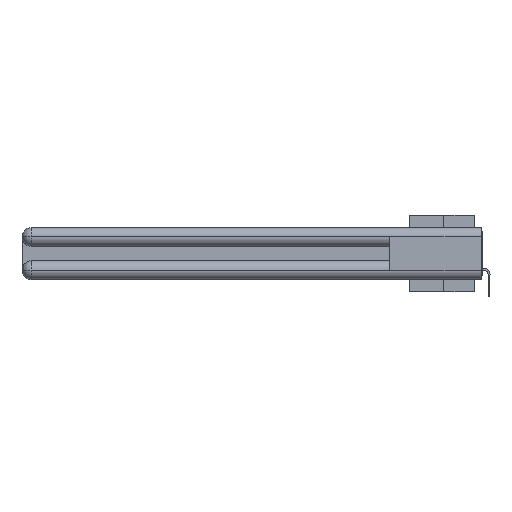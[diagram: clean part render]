
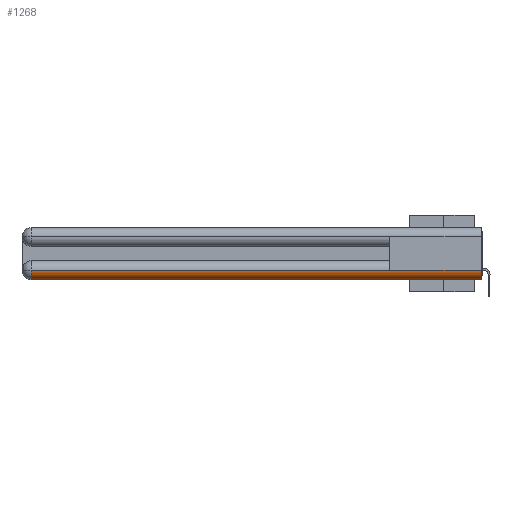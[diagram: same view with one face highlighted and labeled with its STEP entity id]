
A CAD part, left-side view. The second image highlights one B-rep face of the part: STEP entity #1268.
In plain terms, the highlighted cylindrical face has radius 1.562 mm (diameter 3.124 mm), a partial arc.
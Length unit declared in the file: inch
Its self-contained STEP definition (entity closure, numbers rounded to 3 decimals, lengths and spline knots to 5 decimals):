
#1268 = ADVANCED_FACE ( 'NONE', ( #8124 ), #1566, .T. ) ;
#1288 = CARTESIAN_POINT ( 'NONE',  ( 0.0615, 0., -0.2785 ) ) ;
#1566 = CYLINDRICAL_SURFACE ( 'NONE', #31133, 0.0615 ) ;
#2992 = ORIENTED_EDGE ( 'NONE', *, *, #8894, .F. ) ;
#3281 = VERTEX_POINT ( 'NONE', #24042 ) ;
#3698 = CARTESIAN_POINT ( 'NONE',  ( 0.0615, 0., -0.2785 ) ) ;
#6076 = DIRECTION ( 'NONE',  ( 0., 0., 1. ) ) ;
#6688 = DIRECTION ( 'NONE',  ( 0., 1., 0. ) ) ;
#6806 = CIRCLE ( 'NONE', #15072, 0.0615 ) ;
#7131 = VECTOR ( 'NONE', #18733, 39.37008 ) ;
#7229 = CARTESIAN_POINT ( 'NONE',  ( 0., 0., -0.2785 ) ) ;
#8047 = CARTESIAN_POINT ( 'NONE',  ( 0.0615, 0., -0.34 ) ) ;
#8124 = FACE_OUTER_BOUND ( 'NONE', #14798, .T. ) ;
#8366 = LINE ( 'NONE', #31114, #16164 ) ;
#8560 = DIRECTION ( 'NONE',  ( 1., 0., 0. ) ) ;
#8857 = DIRECTION ( 'NONE',  ( 0., 0., -1. ) ) ;
#8894 = EDGE_CURVE ( 'NONE', #30021, #3281, #8366, .T. ) ;
#9548 = VERTEX_POINT ( 'NONE', #7229 ) ;
#10403 = LINE ( 'NONE', #26552, #30623 ) ;
#10723 = CARTESIAN_POINT ( 'NONE',  ( 0., 2.94, -0.2785 ) ) ;
#11939 = CARTESIAN_POINT ( 'NONE',  ( 0., 0.6, -0.2785 ) ) ;
#12993 = VERTEX_POINT ( 'NONE', #11939 ) ;
#13615 = DIRECTION ( 'NONE',  ( 0., -1., 0. ) ) ;
#14179 = DIRECTION ( 'NONE',  ( 0., -1., 0. ) ) ;
#14418 = DIRECTION ( 'NONE',  ( 0., 1., 0. ) ) ;
#14798 = EDGE_LOOP ( 'NONE', ( #20279, #30181, #2992, #20172, #18132 ) ) ;
#15072 = AXIS2_PLACEMENT_3D ( 'NONE', #26864, #14179, #6076 ) ;
#15336 = EDGE_CURVE ( 'NONE', #12993, #15503, #10403, .T. ) ;
#15503 = VERTEX_POINT ( 'NONE', #10723 ) ;
#16164 = VECTOR ( 'NONE', #6688, 39.37008 ) ;
#18132 = ORIENTED_EDGE ( 'NONE', *, *, #27125, .F. ) ;
#18733 = DIRECTION ( 'NONE',  ( 0., -1., 0. ) ) ;
#19943 = LINE ( 'NONE', #26480, #7131 ) ;
#20172 = ORIENTED_EDGE ( 'NONE', *, *, #20802, .F. ) ;
#20261 = AXIS2_PLACEMENT_3D ( 'NONE', #3698, #29005, #8560 ) ;
#20279 = ORIENTED_EDGE ( 'NONE', *, *, #15336, .T. ) ;
#20800 = EDGE_CURVE ( 'NONE', #15503, #3281, #6806, .T. ) ;
#20802 = EDGE_CURVE ( 'NONE', #9548, #30021, #30868, .T. ) ;
#24042 = CARTESIAN_POINT ( 'NONE',  ( 0.0615, 2.94, -0.34 ) ) ;
#26480 = CARTESIAN_POINT ( 'NONE',  ( 0., 0., -0.2785 ) ) ;
#26552 = CARTESIAN_POINT ( 'NONE',  ( 0., 0., -0.2785 ) ) ;
#26864 = CARTESIAN_POINT ( 'NONE',  ( 0.0615, 2.94, -0.2785 ) ) ;
#27125 = EDGE_CURVE ( 'NONE', #12993, #9548, #19943, .T. ) ;
#29005 = DIRECTION ( 'NONE',  ( 0., -1., 0. ) ) ;
#30021 = VERTEX_POINT ( 'NONE', #8047 ) ;
#30181 = ORIENTED_EDGE ( 'NONE', *, *, #20800, .T. ) ;
#30623 = VECTOR ( 'NONE', #14418, 39.37008 ) ;
#30868 = CIRCLE ( 'NONE', #20261, 0.0615 ) ;
#31114 = CARTESIAN_POINT ( 'NONE',  ( 0.0615, 0., -0.34 ) ) ;
#31133 = AXIS2_PLACEMENT_3D ( 'NONE', #1288, #13615, #8857 ) ;
